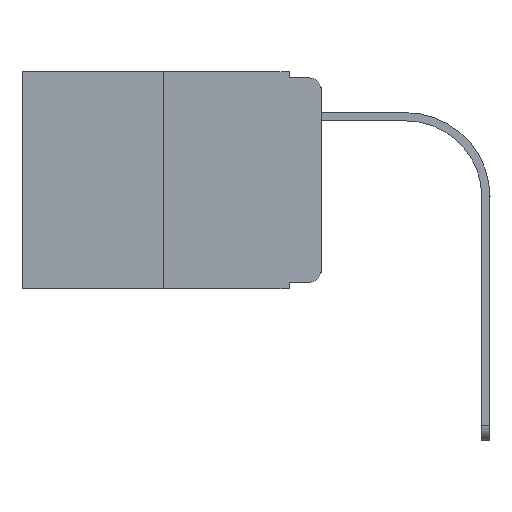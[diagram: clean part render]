
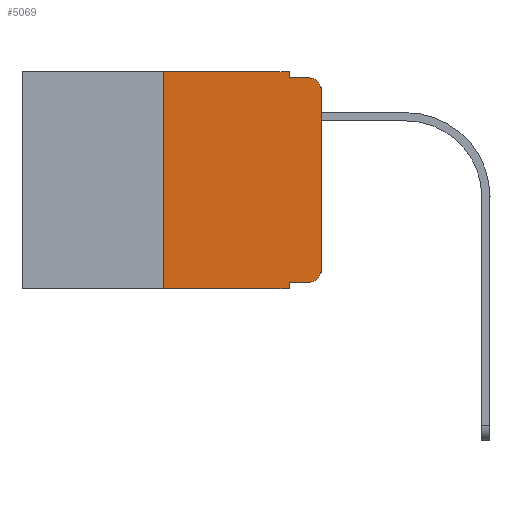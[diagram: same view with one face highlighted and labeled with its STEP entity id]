
A CAD part, left-side view. The second image highlights one B-rep face of the part: STEP entity #5069.
In plain terms, the highlighted planar face has unit normal (-1, 0, 0).
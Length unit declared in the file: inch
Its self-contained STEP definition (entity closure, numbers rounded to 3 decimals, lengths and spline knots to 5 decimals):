
#1031 = VERTEX_POINT ( 'NONE', #4272 ) ;
#1592 = EDGE_CURVE ( 'NONE', #17419, #4031, #8854, .T. ) ;
#2693 = LINE ( 'NONE', #8651, #24712 ) ;
#2787 = LINE ( 'NONE', #15127, #24631 ) ;
#3595 = ORIENTED_EDGE ( 'NONE', *, *, #6374, .T. ) ;
#3713 = ORIENTED_EDGE ( 'NONE', *, *, #4716, .F. ) ;
#3742 = CARTESIAN_POINT ( 'NONE',  ( 0., 0.051, 0. ) ) ;
#3932 = VECTOR ( 'NONE', #23985, 39.37008 ) ;
#4031 = VERTEX_POINT ( 'NONE', #22259 ) ;
#4144 = DIRECTION ( 'NONE',  ( -1., 0., 0. ) ) ;
#4230 = CARTESIAN_POINT ( 'NONE',  ( 0., 0.051, 0. ) ) ;
#4272 = CARTESIAN_POINT ( 'NONE',  ( 0., 0.02, -0.333 ) ) ;
#4342 = AXIS2_PLACEMENT_3D ( 'NONE', #16941, #22833, #18674 ) ;
#4716 = EDGE_CURVE ( 'NONE', #4031, #6575, #2787, .T. ) ;
#5069 = ADVANCED_FACE ( 'NONE', ( #11801 ), #22962, .F. ) ;
#5597 = LINE ( 'NONE', #3742, #19641 ) ;
#6167 = VERTEX_POINT ( 'NONE', #21333 ) ;
#6374 = EDGE_CURVE ( 'NONE', #17419, #19459, #18498, .T. ) ;
#6575 = VERTEX_POINT ( 'NONE', #25425 ) ;
#6591 = CARTESIAN_POINT ( 'NONE',  ( 0., 0.02, -0.03 ) ) ;
#6640 = ORIENTED_EDGE ( 'NONE', *, *, #15498, .F. ) ;
#6695 = EDGE_CURVE ( 'NONE', #6575, #6167, #5597, .T. ) ;
#6780 = CIRCLE ( 'NONE', #10173, 0.02 ) ;
#8165 = EDGE_CURVE ( 'NONE', #1031, #10934, #6780, .T. ) ;
#8493 = DIRECTION ( 'NONE',  ( 0., 0., -1. ) ) ;
#8515 = CARTESIAN_POINT ( 'NONE',  ( 0., 0., -0.03 ) ) ;
#8651 = CARTESIAN_POINT ( 'NONE',  ( 0., 0.051, -0.333 ) ) ;
#8854 = LINE ( 'NONE', #24994, #11027 ) ;
#8981 = CARTESIAN_POINT ( 'NONE',  ( 0., 0.051, -0.01 ) ) ;
#10173 = AXIS2_PLACEMENT_3D ( 'NONE', #24891, #4144, #8493 ) ;
#10934 = VERTEX_POINT ( 'NONE', #24919 ) ;
#11027 = VECTOR ( 'NONE', #18846, 39.37008 ) ;
#11801 = FACE_OUTER_BOUND ( 'NONE', #25882, .T. ) ;
#11918 = EDGE_CURVE ( 'NONE', #6167, #13042, #18961, .T. ) ;
#11950 = ORIENTED_EDGE ( 'NONE', *, *, #26263, .T. ) ;
#13042 = VERTEX_POINT ( 'NONE', #13831 ) ;
#13525 = EDGE_CURVE ( 'NONE', #22884, #1031, #2693, .T. ) ;
#13831 = CARTESIAN_POINT ( 'NONE',  ( 0., 0.02, -0.01 ) ) ;
#14095 = ORIENTED_EDGE ( 'NONE', *, *, #11918, .F. ) ;
#14700 = DIRECTION ( 'NONE',  ( 0., 0., -1. ) ) ;
#14927 = VECTOR ( 'NONE', #22512, 39.37008 ) ;
#15127 = CARTESIAN_POINT ( 'NONE',  ( 0., 0.473, 0. ) ) ;
#15350 = CARTESIAN_POINT ( 'NONE',  ( 0., 0.051, -0.343 ) ) ;
#15498 = EDGE_CURVE ( 'NONE', #22884, #19459, #16180, .T. ) ;
#15693 = ORIENTED_EDGE ( 'NONE', *, *, #1592, .F. ) ;
#16155 = EDGE_CURVE ( 'NONE', #10934, #21788, #22104, .T. ) ;
#16180 = LINE ( 'NONE', #4230, #19167 ) ;
#16941 = CARTESIAN_POINT ( 'NONE',  ( 0., 0.473, 0. ) ) ;
#17419 = VERTEX_POINT ( 'NONE', #19059 ) ;
#17872 = ORIENTED_EDGE ( 'NONE', *, *, #6695, .F. ) ;
#18498 = LINE ( 'NONE', #24646, #14927 ) ;
#18674 = DIRECTION ( 'NONE',  ( 0., 0., -1. ) ) ;
#18846 = DIRECTION ( 'NONE',  ( 0., 0., 1. ) ) ;
#18961 = LINE ( 'NONE', #8981, #26113 ) ;
#18976 = DIRECTION ( 'NONE',  ( 0., -1., 0. ) ) ;
#19059 = CARTESIAN_POINT ( 'NONE',  ( 0., 0.25, -0.343 ) ) ;
#19167 = VECTOR ( 'NONE', #20322, 39.37008 ) ;
#19289 = DIRECTION ( 'NONE',  ( 0., -1., 0. ) ) ;
#19459 = VERTEX_POINT ( 'NONE', #15350 ) ;
#19641 = VECTOR ( 'NONE', #20089, 39.37008 ) ;
#20089 = DIRECTION ( 'NONE',  ( 0., 0., -1. ) ) ;
#20322 = DIRECTION ( 'NONE',  ( 0., 0., -1. ) ) ;
#21333 = CARTESIAN_POINT ( 'NONE',  ( 0., 0.051, -0.01 ) ) ;
#21400 = CIRCLE ( 'NONE', #23534, 0.02 ) ;
#21788 = VERTEX_POINT ( 'NONE', #8515 ) ;
#21907 = ORIENTED_EDGE ( 'NONE', *, *, #13525, .T. ) ;
#22104 = LINE ( 'NONE', #24237, #3932 ) ;
#22128 = CARTESIAN_POINT ( 'NONE',  ( 0., 0.051, -0.333 ) ) ;
#22259 = CARTESIAN_POINT ( 'NONE',  ( 0., 0.25, 0. ) ) ;
#22512 = DIRECTION ( 'NONE',  ( 0., -1., 0. ) ) ;
#22827 = DIRECTION ( 'NONE',  ( -1., 0., 0. ) ) ;
#22833 = DIRECTION ( 'NONE',  ( 1., 0., 0. ) ) ;
#22884 = VERTEX_POINT ( 'NONE', #22128 ) ;
#22962 = PLANE ( 'NONE',  #4342 ) ;
#23534 = AXIS2_PLACEMENT_3D ( 'NONE', #6591, #22827, #14700 ) ;
#23985 = DIRECTION ( 'NONE',  ( 0., 0., 1. ) ) ;
#24237 = CARTESIAN_POINT ( 'NONE',  ( 0., 0., 0. ) ) ;
#24286 = ORIENTED_EDGE ( 'NONE', *, *, #16155, .T. ) ;
#24631 = VECTOR ( 'NONE', #18976, 39.37008 ) ;
#24646 = CARTESIAN_POINT ( 'NONE',  ( 0., 0.473, -0.343 ) ) ;
#24712 = VECTOR ( 'NONE', #19289, 39.37008 ) ;
#24891 = CARTESIAN_POINT ( 'NONE',  ( 0., 0.02, -0.313 ) ) ;
#24919 = CARTESIAN_POINT ( 'NONE',  ( 0., 0., -0.313 ) ) ;
#24994 = CARTESIAN_POINT ( 'NONE',  ( 0., 0.25, 0. ) ) ;
#25371 = DIRECTION ( 'NONE',  ( 0., -1., 0. ) ) ;
#25425 = CARTESIAN_POINT ( 'NONE',  ( 0., 0.051, 0. ) ) ;
#25882 = EDGE_LOOP ( 'NONE', ( #24286, #11950, #14095, #17872, #3713, #15693, #3595, #6640, #21907, #26205 ) ) ;
#26113 = VECTOR ( 'NONE', #25371, 39.37008 ) ;
#26205 = ORIENTED_EDGE ( 'NONE', *, *, #8165, .T. ) ;
#26263 = EDGE_CURVE ( 'NONE', #21788, #13042, #21400, .T. ) ;
